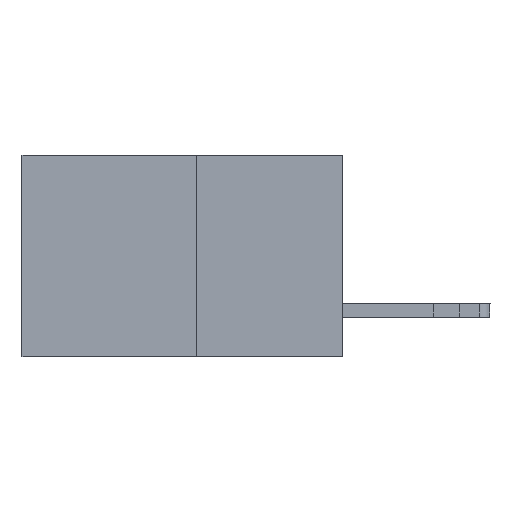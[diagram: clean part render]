
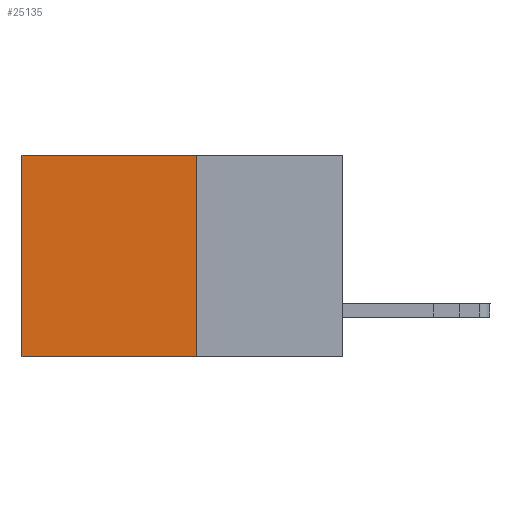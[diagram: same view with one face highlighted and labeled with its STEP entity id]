
A CAD part, left-side view. The second image highlights one B-rep face of the part: STEP entity #25135.
In plain terms, the highlighted planar face has unit normal (-1, 0, 0).
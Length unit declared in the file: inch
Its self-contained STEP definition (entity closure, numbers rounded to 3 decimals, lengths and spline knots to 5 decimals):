
#572 = FACE_OUTER_BOUND ( 'NONE', #21692, .T. ) ;
#894 = DIRECTION ( 'NONE',  ( 0., 0., -1. ) ) ;
#931 = CARTESIAN_POINT ( 'NONE',  ( 0.277, 0.27, 0. ) ) ;
#1976 = CARTESIAN_POINT ( 'NONE',  ( 0.277, 0.27, -0.37 ) ) ;
#4088 = DIRECTION ( 'NONE',  ( 0., 0., -1. ) ) ;
#4316 = CARTESIAN_POINT ( 'NONE',  ( 0.277, 0.59, 0. ) ) ;
#4684 = ORIENTED_EDGE ( 'NONE', *, *, #17698, .T. ) ;
#5582 = CARTESIAN_POINT ( 'NONE',  ( 0.277, 0.27, 0. ) ) ;
#5585 = ORIENTED_EDGE ( 'NONE', *, *, #24000, .F. ) ;
#5775 = DIRECTION ( 'NONE',  ( 0., 1., 0. ) ) ;
#5946 = DIRECTION ( 'NONE',  ( 0., 0., -1. ) ) ;
#7837 = ORIENTED_EDGE ( 'NONE', *, *, #27406, .T. ) ;
#7885 = CARTESIAN_POINT ( 'NONE',  ( 0.277, 0.59, -0.37 ) ) ;
#8890 = ORIENTED_EDGE ( 'NONE', *, *, #27316, .F. ) ;
#9382 = LINE ( 'NONE', #22691, #26965 ) ;
#9714 = VERTEX_POINT ( 'NONE', #931 ) ;
#9959 = DIRECTION ( 'NONE',  ( 0., 1., 0. ) ) ;
#11295 = VERTEX_POINT ( 'NONE', #4316 ) ;
#12029 = LINE ( 'NONE', #5582, #16266 ) ;
#13480 = DIRECTION ( 'NONE',  ( 1., 0., 0. ) ) ;
#14108 = LINE ( 'NONE', #1976, #24835 ) ;
#16072 = VERTEX_POINT ( 'NONE', #19537 ) ;
#16266 = VECTOR ( 'NONE', #5775, 39.37008 ) ;
#16453 = CARTESIAN_POINT ( 'NONE',  ( 0.277, 0.59, -0.37 ) ) ;
#17698 = EDGE_CURVE ( 'NONE', #9714, #11295, #12029, .T. ) ;
#17839 = AXIS2_PLACEMENT_3D ( 'NONE', #19807, #13480, #894 ) ;
#17926 = VECTOR ( 'NONE', #5946, 39.37008 ) ;
#19537 = CARTESIAN_POINT ( 'NONE',  ( 0.277, 0.27, -0.37 ) ) ;
#19807 = CARTESIAN_POINT ( 'NONE',  ( 0.277, 0.27, -0.37 ) ) ;
#21261 = VERTEX_POINT ( 'NONE', #7885 ) ;
#21692 = EDGE_LOOP ( 'NONE', ( #7837, #8890, #5585, #4684 ) ) ;
#22691 = CARTESIAN_POINT ( 'NONE',  ( 0.277, 0.27, -0.37 ) ) ;
#24000 = EDGE_CURVE ( 'NONE', #9714, #16072, #14108, .T. ) ;
#24324 = LINE ( 'NONE', #16453, #17926 ) ;
#24835 = VECTOR ( 'NONE', #4088, 39.37008 ) ;
#25135 = ADVANCED_FACE ( 'NONE', ( #572 ), #26284, .F. ) ;
#26284 = PLANE ( 'NONE',  #17839 ) ;
#26965 = VECTOR ( 'NONE', #9959, 39.37008 ) ;
#27316 = EDGE_CURVE ( 'NONE', #16072, #21261, #9382, .T. ) ;
#27406 = EDGE_CURVE ( 'NONE', #11295, #21261, #24324, .T. ) ;
